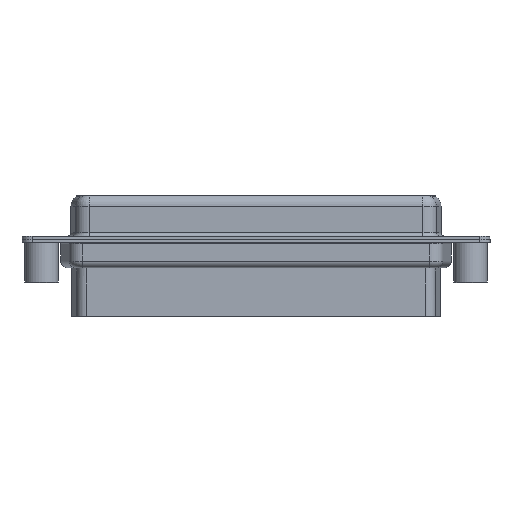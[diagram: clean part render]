
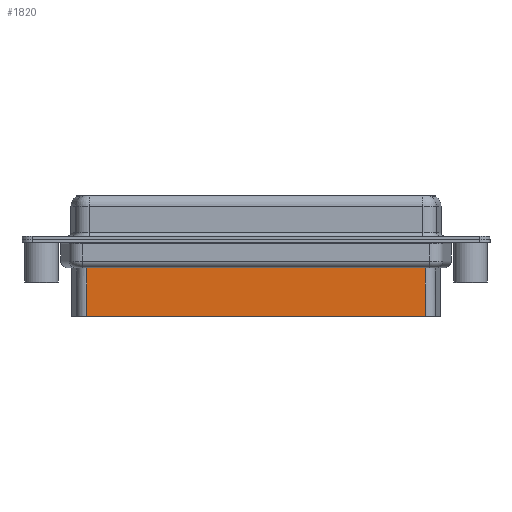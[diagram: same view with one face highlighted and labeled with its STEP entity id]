
A CAD part, front view. The second image highlights one B-rep face of the part: STEP entity #1820.
In plain terms, the highlighted planar face has unit normal (0, -1, 0).
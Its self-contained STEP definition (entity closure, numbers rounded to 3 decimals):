
#410 = LINE ( 'NONE', #21400, #13139 ) ;
#492 = CARTESIAN_POINT ( 'NONE',  ( 6.706, -3.5, -4.097 ) ) ;
#615 = DIRECTION ( 'NONE',  ( -1., 0., 0. ) ) ;
#1820 = ADVANCED_FACE ( 'NONE', ( #22532 ), #20521, .T. ) ;
#2340 = VERTEX_POINT ( 'NONE', #492 ) ;
#2871 = LINE ( 'NONE', #8560, #16693 ) ;
#2908 = ORIENTED_EDGE ( 'NONE', *, *, #3490, .T. ) ;
#3490 = EDGE_CURVE ( 'NONE', #2340, #10411, #17683, .T. ) ;
#7110 = EDGE_CURVE ( 'NONE', #20939, #2340, #410, .T. ) ;
#7912 = EDGE_CURVE ( 'NONE', #9166, #10411, #18145, .T. ) ;
#8057 = CARTESIAN_POINT ( 'NONE',  ( 56.794, -3.5, -4.097 ) ) ;
#8530 = ORIENTED_EDGE ( 'NONE', *, *, #8747, .F. ) ;
#8560 = CARTESIAN_POINT ( 'NONE',  ( 56.794, -3.5, -3.1 ) ) ;
#8747 = EDGE_CURVE ( 'NONE', #20939, #9166, #2871, .T. ) ;
#9150 = VECTOR ( 'NONE', #615, 1000. ) ;
#9166 = VERTEX_POINT ( 'NONE', #14959 ) ;
#9715 = CARTESIAN_POINT ( 'NONE',  ( 6.706, -3.5, -11.45 ) ) ;
#10396 = ORIENTED_EDGE ( 'NONE', *, *, #7110, .T. ) ;
#10411 = VERTEX_POINT ( 'NONE', #17467 ) ;
#10661 = DIRECTION ( 'NONE',  ( -1., 0., 0. ) ) ;
#12204 = AXIS2_PLACEMENT_3D ( 'NONE', #20593, #18660, #18522 ) ;
#13139 = VECTOR ( 'NONE', #10661, 1000. ) ;
#14272 = ORIENTED_EDGE ( 'NONE', *, *, #7912, .F. ) ;
#14959 = CARTESIAN_POINT ( 'NONE',  ( 56.794, -3.5, -11.45 ) ) ;
#16693 = VECTOR ( 'NONE', #21125, 1000. ) ;
#17122 = VECTOR ( 'NONE', #21977, 1000. ) ;
#17467 = CARTESIAN_POINT ( 'NONE',  ( 6.706, -3.5, -11.45 ) ) ;
#17683 = LINE ( 'NONE', #22047, #17122 ) ;
#18145 = LINE ( 'NONE', #9715, #9150 ) ;
#18522 = DIRECTION ( 'NONE',  ( 1., 0., 0. ) ) ;
#18660 = DIRECTION ( 'NONE',  ( 0., -1., 0. ) ) ;
#20521 = PLANE ( 'NONE',  #12204 ) ;
#20593 = CARTESIAN_POINT ( 'NONE',  ( 6.706, -3.5, -3.1 ) ) ;
#20939 = VERTEX_POINT ( 'NONE', #8057 ) ;
#21125 = DIRECTION ( 'NONE',  ( 0., 0., -1. ) ) ;
#21400 = CARTESIAN_POINT ( 'NONE',  ( 6.459, -3.5, -4.097 ) ) ;
#21977 = DIRECTION ( 'NONE',  ( 0., 0., -1. ) ) ;
#22047 = CARTESIAN_POINT ( 'NONE',  ( 6.706, -3.5, -3.1 ) ) ;
#22532 = FACE_OUTER_BOUND ( 'NONE', #22965, .T. ) ;
#22965 = EDGE_LOOP ( 'NONE', ( #8530, #10396, #2908, #14272 ) ) ;
